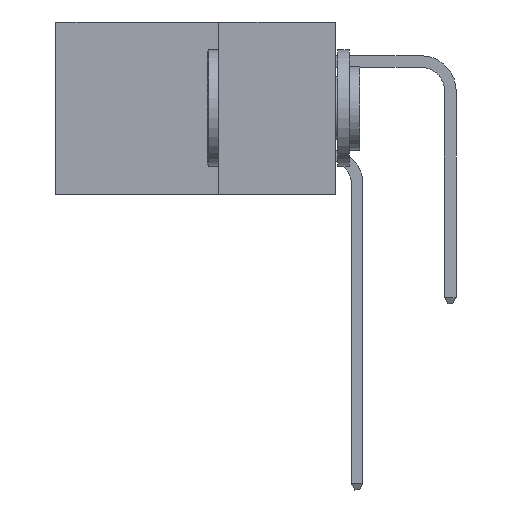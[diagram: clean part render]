
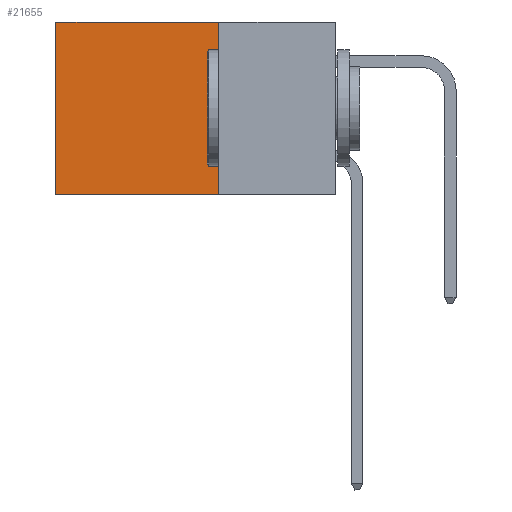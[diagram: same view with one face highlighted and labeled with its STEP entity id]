
A CAD part, left-side view. The second image highlights one B-rep face of the part: STEP entity #21655.
In plain terms, the highlighted planar face has unit normal (-1, 0, 0).
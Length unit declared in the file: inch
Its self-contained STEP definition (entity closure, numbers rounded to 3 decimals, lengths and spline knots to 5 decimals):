
#920 = DIRECTION ( 'NONE',  ( 0., 1., 0. ) ) ;
#952 = LINE ( 'NONE', #30656, #16126 ) ;
#1367 = CARTESIAN_POINT ( 'NONE',  ( 0.2875, 0.25, 0. ) ) ;
#2699 = ORIENTED_EDGE ( 'NONE', *, *, #39872, .F. ) ;
#3336 = EDGE_LOOP ( 'NONE', ( #21740, #2699, #36048, #40455 ) ) ;
#5395 = EDGE_CURVE ( 'NONE', #31065, #34494, #38607, .T. ) ;
#6398 = CARTESIAN_POINT ( 'NONE',  ( 0.2875, 0.25, -0.37 ) ) ;
#6751 = LINE ( 'NONE', #12658, #25980 ) ;
#7216 = CARTESIAN_POINT ( 'NONE',  ( 0.2875, 0.6, -0.37 ) ) ;
#7619 = VERTEX_POINT ( 'NONE', #6398 ) ;
#10489 = VERTEX_POINT ( 'NONE', #7216 ) ;
#12658 = CARTESIAN_POINT ( 'NONE',  ( 0.2875, 0.6, 0. ) ) ;
#12710 = EDGE_CURVE ( 'NONE', #34494, #10489, #6751, .T. ) ;
#14185 = DIRECTION ( 'NONE',  ( 0., 0., -1. ) ) ;
#15709 = DIRECTION ( 'NONE',  ( 0., 0., -1. ) ) ;
#16126 = VECTOR ( 'NONE', #920, 39.37008 ) ;
#18353 = FACE_OUTER_BOUND ( 'NONE', #3336, .T. ) ;
#18843 = DIRECTION ( 'NONE',  ( 1., 0., 0. ) ) ;
#19008 = LINE ( 'NONE', #1367, #41729 ) ;
#19997 = CARTESIAN_POINT ( 'NONE',  ( 0.2875, 0.25, 0. ) ) ;
#21655 = ADVANCED_FACE ( 'NONE', ( #18353 ), #22486, .F. ) ;
#21740 = ORIENTED_EDGE ( 'NONE', *, *, #12710, .T. ) ;
#21827 = CARTESIAN_POINT ( 'NONE',  ( 0.2875, 0.25, 0. ) ) ;
#22486 = PLANE ( 'NONE',  #30779 ) ;
#22688 = CARTESIAN_POINT ( 'NONE',  ( 0.2875, 0.6, 0. ) ) ;
#25980 = VECTOR ( 'NONE', #33572, 39.37008 ) ;
#26134 = EDGE_CURVE ( 'NONE', #31065, #7619, #19008, .T. ) ;
#28587 = DIRECTION ( 'NONE',  ( 0., 1., 0. ) ) ;
#30056 = VECTOR ( 'NONE', #28587, 39.37008 ) ;
#30656 = CARTESIAN_POINT ( 'NONE',  ( 0.2875, 0.25, -0.37 ) ) ;
#30779 = AXIS2_PLACEMENT_3D ( 'NONE', #37485, #18843, #15709 ) ;
#31065 = VERTEX_POINT ( 'NONE', #19997 ) ;
#33572 = DIRECTION ( 'NONE',  ( 0., 0., -1. ) ) ;
#34494 = VERTEX_POINT ( 'NONE', #22688 ) ;
#36048 = ORIENTED_EDGE ( 'NONE', *, *, #26134, .F. ) ;
#37485 = CARTESIAN_POINT ( 'NONE',  ( 0.2875, 0.25, 0. ) ) ;
#38607 = LINE ( 'NONE', #21827, #30056 ) ;
#39872 = EDGE_CURVE ( 'NONE', #7619, #10489, #952, .T. ) ;
#40455 = ORIENTED_EDGE ( 'NONE', *, *, #5395, .T. ) ;
#41729 = VECTOR ( 'NONE', #14185, 39.37008 ) ;
